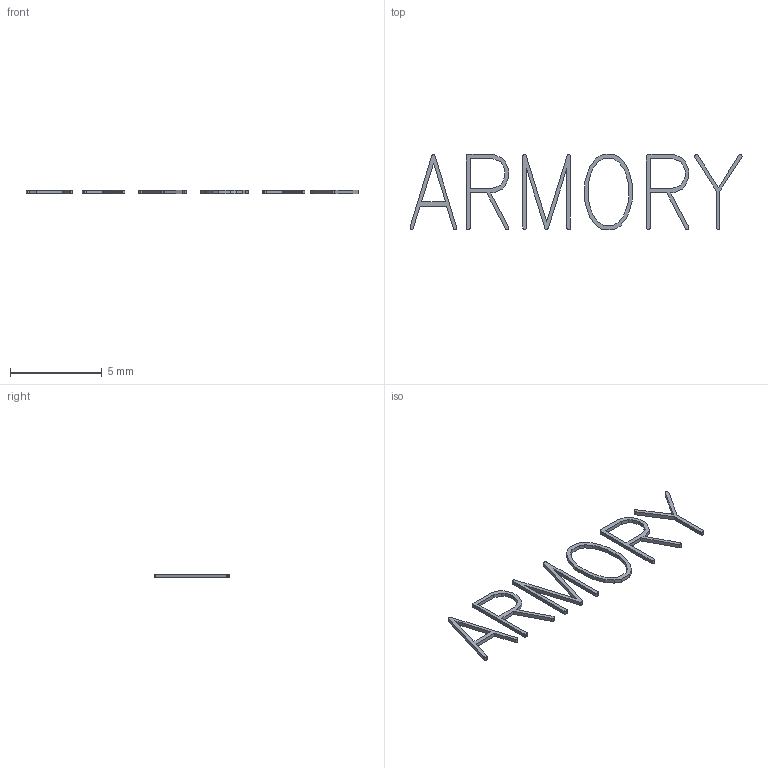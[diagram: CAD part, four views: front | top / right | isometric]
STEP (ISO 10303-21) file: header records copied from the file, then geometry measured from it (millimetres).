
FILE_DESCRIPTION (( 'STEP AP214' ), '1' );
FILE_NAME ('ENGRAVING FILL - ARMORY.STEP', '2013-06-19T14:05:48', ( 'Asher' ), ( '' ), 'SwSTEP 2.0', 'SolidWorks 2013', '' );
FILE_SCHEMA (( 'AUTOMOTIVE_DESIGN' ));
Length unit declared in the file: millimetre
Products named in the file (1): ENGRAVING FILL - ARMORY
Bounding box: 18.11 x 4.11 x 0.2 mm (x, y, z)
Volume: 2.7 mm3; surface area: 52.4 mm2
Topology: 6 solids, 6 shells, 176 faces, 492 edges, 328 vertices
Faces by surface type: plane 127, bspline 49
Entity records: 6433 total; most frequent: CARTESIAN_POINT 2142, ORIENTED_EDGE 984, DIRECTION 650, EDGE_CURVE 492, LINE 394, VECTOR 394, VERTEX_POINT 328, EDGE_LOOP 184
